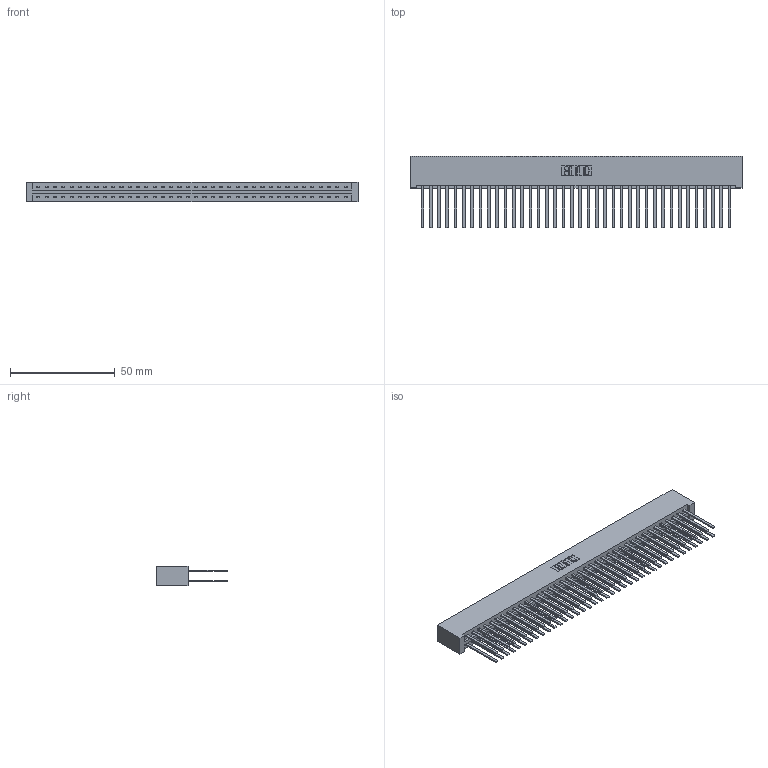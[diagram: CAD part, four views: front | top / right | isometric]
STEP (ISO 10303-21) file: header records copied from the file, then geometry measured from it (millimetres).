
FILE_DESCRIPTION (( 'STEP AP203' ), '1' );
FILE_NAME ('337-076-544-201.STEP', '2019-10-10T10:46:05', ( '' ), ( '' ), 'SwSTEP 2.0', 'SolidWorks 2016', '' );
FILE_SCHEMA (( 'CONFIG_CONTROL_DESIGN' ));
Length unit declared in the file: inch
Products named in the file (3): 337-076-544-201; 337 Part_No Mounting Lugs; 345-292-001_345-293-144
Assembly tree (77 placements, depth 2):
  337-076-544-201
    337 Part_No Mounting Lugs
    345-292-001_345-293-144  x76
Bounding box: 158.45 x 34.3 x 9.4 mm (x, y, z)
Volume: 18471.1 mm3; surface area: 24379.2 mm2
Topology: 77 solids, 77 shells, 3754 faces, 11155 edges, 7334 vertices
Faces by surface type: plane 2650, cylinder 1104
Entity records: 29519 total; most frequent: CARTESIAN_POINT 4974, ORIENTED_EDGE 4910, DIRECTION 4227, EDGE_CURVE 2455, VECTOR 2339, LINE 2339, VERTEX_POINT 1634, AXIS2_PLACEMENT_3D 944
